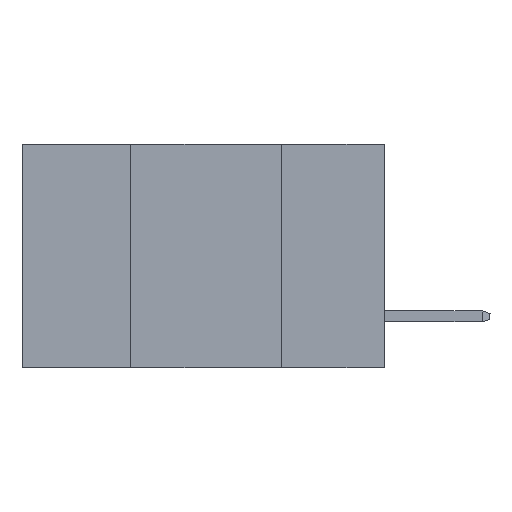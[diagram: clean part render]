
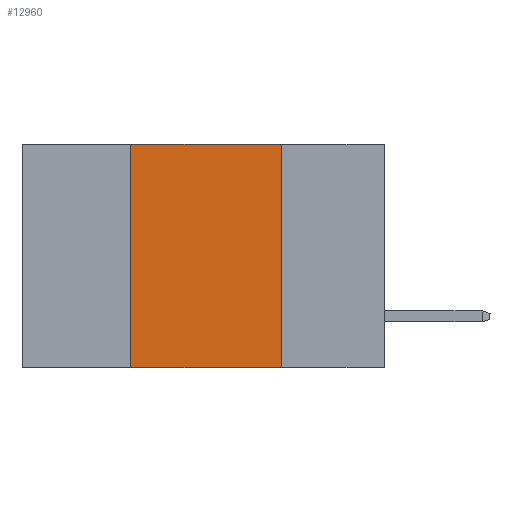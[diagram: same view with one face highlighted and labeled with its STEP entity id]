
A CAD part, left-side view. The second image highlights one B-rep face of the part: STEP entity #12960.
In plain terms, the highlighted planar face has unit normal (-1, 0, 0).
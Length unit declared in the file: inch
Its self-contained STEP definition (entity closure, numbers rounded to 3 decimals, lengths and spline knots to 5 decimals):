
#284 = AXIS2_PLACEMENT_3D ( 'NONE', #1434, #5998, #1587 ) ;
#304 = CARTESIAN_POINT ( 'NONE',  ( 0., 0.17, 0. ) ) ;
#792 = VECTOR ( 'NONE', #4756, 39.37008 ) ;
#807 = CARTESIAN_POINT ( 'NONE',  ( 0., 0.42, -0.37 ) ) ;
#1323 = LINE ( 'NONE', #10457, #792 ) ;
#1434 = CARTESIAN_POINT ( 'NONE',  ( 0., 0.6, 0. ) ) ;
#1587 = DIRECTION ( 'NONE',  ( 0., 0., -1. ) ) ;
#1792 = LINE ( 'NONE', #807, #13102 ) ;
#2324 = DIRECTION ( 'NONE',  ( 0., -1., 0. ) ) ;
#2605 = VECTOR ( 'NONE', #5341, 39.37008 ) ;
#4183 = DIRECTION ( 'NONE',  ( 0., 0., 1. ) ) ;
#4206 = ORIENTED_EDGE ( 'NONE', *, *, #7869, .F. ) ;
#4756 = DIRECTION ( 'NONE',  ( 0., 0., -1. ) ) ;
#5268 = LINE ( 'NONE', #8855, #2605 ) ;
#5341 = DIRECTION ( 'NONE',  ( 0., -1., 0. ) ) ;
#5463 = ORIENTED_EDGE ( 'NONE', *, *, #10342, .F. ) ;
#5534 = ORIENTED_EDGE ( 'NONE', *, *, #13602, .F. ) ;
#5947 = VERTEX_POINT ( 'NONE', #304 ) ;
#5998 = DIRECTION ( 'NONE',  ( 1., 0., 0. ) ) ;
#6904 = VERTEX_POINT ( 'NONE', #14478 ) ;
#7547 = VECTOR ( 'NONE', #2324, 39.37008 ) ;
#7869 = EDGE_CURVE ( 'NONE', #8854, #10100, #1792, .T. ) ;
#8854 = VERTEX_POINT ( 'NONE', #12823 ) ;
#8855 = CARTESIAN_POINT ( 'NONE',  ( 0., 0.6, 0. ) ) ;
#9081 = EDGE_CURVE ( 'NONE', #8854, #6904, #13419, .T. ) ;
#10100 = VERTEX_POINT ( 'NONE', #13752 ) ;
#10136 = ORIENTED_EDGE ( 'NONE', *, *, #9081, .T. ) ;
#10342 = EDGE_CURVE ( 'NONE', #10100, #5947, #5268, .T. ) ;
#10457 = CARTESIAN_POINT ( 'NONE',  ( 0., 0.17, -0.37 ) ) ;
#10960 = EDGE_LOOP ( 'NONE', ( #5534, #5463, #4206, #10136 ) ) ;
#11689 = FACE_OUTER_BOUND ( 'NONE', #10960, .T. ) ;
#11841 = PLANE ( 'NONE',  #284 ) ;
#12823 = CARTESIAN_POINT ( 'NONE',  ( 0., 0.42, -0.37 ) ) ;
#12960 = ADVANCED_FACE ( 'NONE', ( #11689 ), #11841, .F. ) ;
#13102 = VECTOR ( 'NONE', #4183, 39.37008 ) ;
#13419 = LINE ( 'NONE', #13568, #7547 ) ;
#13568 = CARTESIAN_POINT ( 'NONE',  ( 0., 0.6, -0.37 ) ) ;
#13602 = EDGE_CURVE ( 'NONE', #5947, #6904, #1323, .T. ) ;
#13752 = CARTESIAN_POINT ( 'NONE',  ( 0., 0.42, 0. ) ) ;
#14478 = CARTESIAN_POINT ( 'NONE',  ( 0., 0.17, -0.37 ) ) ;
